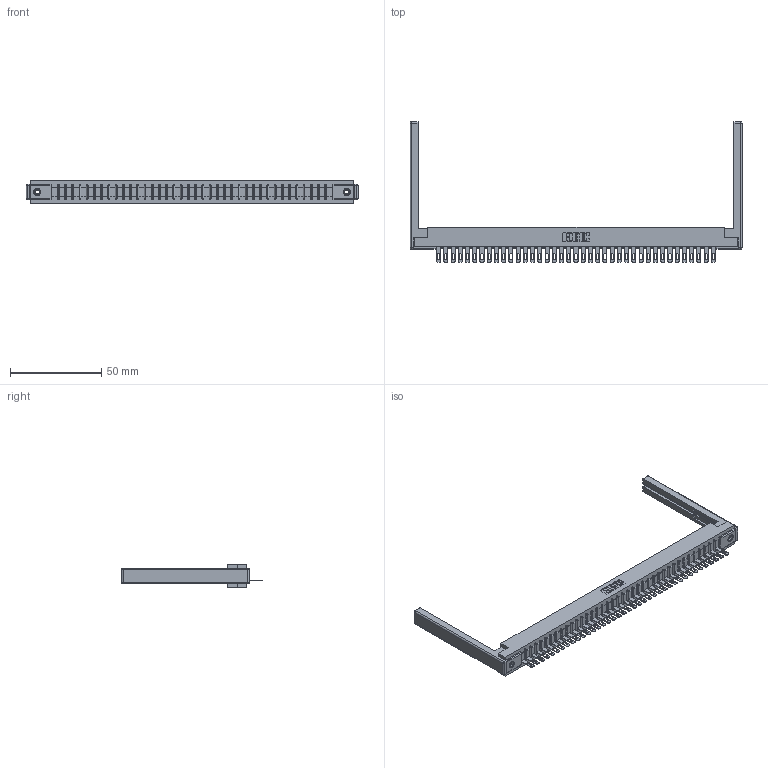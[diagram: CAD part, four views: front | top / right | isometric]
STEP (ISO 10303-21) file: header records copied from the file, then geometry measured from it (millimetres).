
FILE_DESCRIPTION (( 'STEP AP203' ), '1' );
FILE_NAME ('357-039-405-168.STEP', '2020-10-02T22:19:02', ( '' ), ( '' ), 'SwSTEP 2.0', 'SolidWorks 2020', '' );
FILE_SCHEMA (( 'CONFIG_CONTROL_DESIGN' ));
Length unit declared in the file: inch
Products named in the file (5): 345-250-001_345-250-001-102; 307 Part_.156 Dia Mounting Holes; 307-290-001_505; 357-039-405-168; 307-220-068
Assembly tree (44 placements, depth 2):
  357-039-405-168
    307 Part_.156 Dia Mounting Holes
    307-290-001_505  x39
    307-220-068  x2
    345-250-001_345-250-001-102  x2
Bounding box: 181.97 x 77.14 x 12.7 mm (x, y, z)
Volume: 23317.8 mm3; surface area: 24409.5 mm2
Topology: 44 solids, 44 shells, 2496 faces, 7031 edges, 4506 vertices
Faces by surface type: plane 1562, cylinder 830, sphere 88, cone 12, torus 4
Entity records: 36537 total; most frequent: CARTESIAN_POINT 6117, ORIENTED_EDGE 6092, DIRECTION 5970, EDGE_CURVE 3046, VECTOR 2332, LINE 2332, VERTEX_POINT 1966, AXIS2_PLACEMENT_3D 1819
